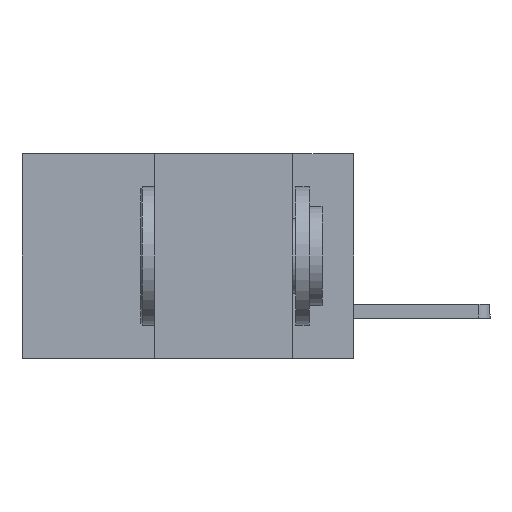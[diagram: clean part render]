
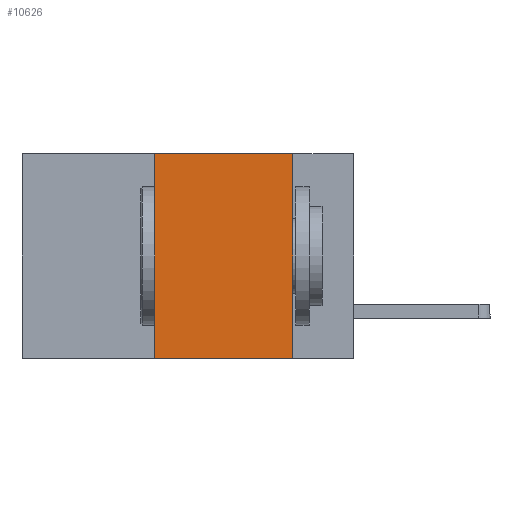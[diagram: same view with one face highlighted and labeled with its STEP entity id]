
A CAD part, left-side view. The second image highlights one B-rep face of the part: STEP entity #10626.
In plain terms, the highlighted planar face has unit normal (-1, 0, 0).
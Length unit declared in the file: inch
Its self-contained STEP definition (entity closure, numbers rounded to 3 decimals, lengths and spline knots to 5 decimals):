
#542 = LINE ( 'NONE', #5093, #4759 ) ;
#635 = ORIENTED_EDGE ( 'NONE', *, *, #7653, .F. ) ;
#752 = ORIENTED_EDGE ( 'NONE', *, *, #7726, .T. ) ;
#775 = CARTESIAN_POINT ( 'NONE',  ( 0., 0.36, 0. ) ) ;
#1088 = LINE ( 'NONE', #9735, #3056 ) ;
#1471 = VERTEX_POINT ( 'NONE', #2733 ) ;
#1534 = LINE ( 'NONE', #2515, #3509 ) ;
#1590 = VERTEX_POINT ( 'NONE', #7371 ) ;
#1680 = VERTEX_POINT ( 'NONE', #3776 ) ;
#2515 = CARTESIAN_POINT ( 'NONE',  ( 0., 0.11, 0. ) ) ;
#2733 = CARTESIAN_POINT ( 'NONE',  ( 0., 0.36, -0.37 ) ) ;
#3056 = VECTOR ( 'NONE', #9828, 39.37008 ) ;
#3090 = EDGE_CURVE ( 'NONE', #5485, #1590, #1088, .T. ) ;
#3509 = VECTOR ( 'NONE', #5855, 39.37008 ) ;
#3559 = LINE ( 'NONE', #775, #5276 ) ;
#3776 = CARTESIAN_POINT ( 'NONE',  ( 0., 0.11, -0.37 ) ) ;
#4183 = PLANE ( 'NONE',  #4619 ) ;
#4619 = AXIS2_PLACEMENT_3D ( 'NONE', #9872, #5054, #10662 ) ;
#4759 = VECTOR ( 'NONE', #5917, 39.37008 ) ;
#5054 = DIRECTION ( 'NONE',  ( 1., 0., 0. ) ) ;
#5093 = CARTESIAN_POINT ( 'NONE',  ( 0., 0.6, -0.37 ) ) ;
#5276 = VECTOR ( 'NONE', #5843, 39.37008 ) ;
#5485 = VERTEX_POINT ( 'NONE', #8662 ) ;
#5843 = DIRECTION ( 'NONE',  ( 0., 0., 1. ) ) ;
#5855 = DIRECTION ( 'NONE',  ( 0., 0., -1. ) ) ;
#5917 = DIRECTION ( 'NONE',  ( 0., -1., 0. ) ) ;
#7371 = CARTESIAN_POINT ( 'NONE',  ( 0., 0.11, 0. ) ) ;
#7653 = EDGE_CURVE ( 'NONE', #1471, #5485, #3559, .T. ) ;
#7726 = EDGE_CURVE ( 'NONE', #1471, #1680, #542, .T. ) ;
#8662 = CARTESIAN_POINT ( 'NONE',  ( 0., 0.36, 0. ) ) ;
#9436 = ORIENTED_EDGE ( 'NONE', *, *, #9934, .F. ) ;
#9645 = ORIENTED_EDGE ( 'NONE', *, *, #3090, .F. ) ;
#9735 = CARTESIAN_POINT ( 'NONE',  ( 0., 0.6, 0. ) ) ;
#9828 = DIRECTION ( 'NONE',  ( 0., -1., 0. ) ) ;
#9872 = CARTESIAN_POINT ( 'NONE',  ( 0., 0.6, 0. ) ) ;
#9925 = EDGE_LOOP ( 'NONE', ( #9436, #9645, #635, #752 ) ) ;
#9934 = EDGE_CURVE ( 'NONE', #1590, #1680, #1534, .T. ) ;
#10005 = FACE_OUTER_BOUND ( 'NONE', #9925, .T. ) ;
#10626 = ADVANCED_FACE ( 'NONE', ( #10005 ), #4183, .F. ) ;
#10662 = DIRECTION ( 'NONE',  ( 0., 0., -1. ) ) ;
